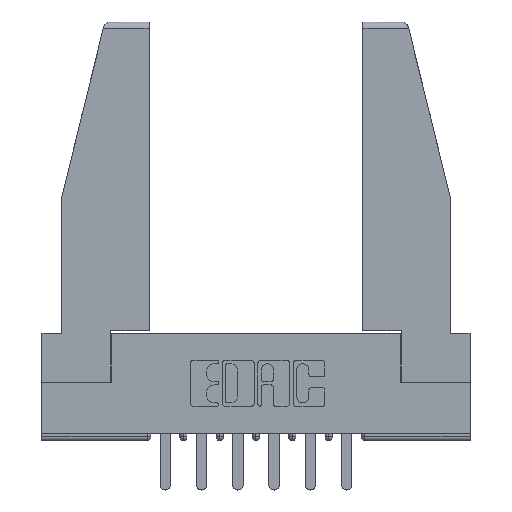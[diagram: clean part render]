
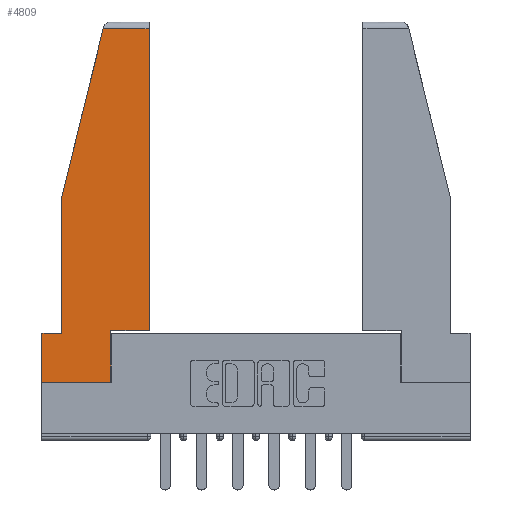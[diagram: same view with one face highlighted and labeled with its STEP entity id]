
A CAD part, top view. The second image highlights one B-rep face of the part: STEP entity #4809.
In plain terms, the highlighted planar face has unit normal (0, 0, 1).
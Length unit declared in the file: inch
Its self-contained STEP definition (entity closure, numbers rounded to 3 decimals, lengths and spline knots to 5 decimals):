
#142 = ORIENTED_EDGE ( 'NONE', *, *, #9193, .T. ) ;
#317 = EDGE_CURVE ( 'NONE', #8245, #10129, #10745, .T. ) ;
#431 = LINE ( 'NONE', #6958, #1872 ) ;
#1487 = VECTOR ( 'NONE', #5805, 39.37008 ) ;
#1565 = CARTESIAN_POINT ( 'NONE',  ( 0.2636, 1.52, 0. ) ) ;
#1872 = VECTOR ( 'NONE', #12044, 39.37008 ) ;
#1889 = VERTEX_POINT ( 'NONE', #7203 ) ;
#1959 = CARTESIAN_POINT ( 'NONE',  ( 0., 0.21, 0. ) ) ;
#2574 = EDGE_CURVE ( 'NONE', #11155, #6368, #4320, .T. ) ;
#2994 = CARTESIAN_POINT ( 'NONE',  ( 0., 0.21, 0. ) ) ;
#3124 = CARTESIAN_POINT ( 'NONE',  ( 0.461, 1.52, 0. ) ) ;
#3129 = CARTESIAN_POINT ( 'NONE',  ( 0., 0., 0. ) ) ;
#3348 = CARTESIAN_POINT ( 'NONE',  ( 0., 0., 0. ) ) ;
#3396 = ORIENTED_EDGE ( 'NONE', *, *, #2574, .T. ) ;
#3424 = EDGE_CURVE ( 'NONE', #10129, #6494, #5858, .T. ) ;
#3546 = CARTESIAN_POINT ( 'NONE',  ( 0., 1.52, 0. ) ) ;
#3784 = CARTESIAN_POINT ( 'NONE',  ( 0.086, 0.8, 0. ) ) ;
#3851 = EDGE_CURVE ( 'NONE', #9938, #8245, #10820, .T. ) ;
#3939 = LINE ( 'NONE', #2994, #7567 ) ;
#3979 = DIRECTION ( 'NONE',  ( 1., 0., 0. ) ) ;
#4041 = DIRECTION ( 'NONE',  ( 0., -1., 0. ) ) ;
#4129 = EDGE_LOOP ( 'NONE', ( #6269, #142, #6934, #8595, #9787, #11433, #3396, #6315, #10667 ) ) ;
#4194 = EDGE_CURVE ( 'NONE', #6368, #1889, #7581, .T. ) ;
#4320 = LINE ( 'NONE', #7460, #12112 ) ;
#4431 = VECTOR ( 'NONE', #6038, 39.37008 ) ;
#4789 = EDGE_CURVE ( 'NONE', #6494, #11155, #3939, .T. ) ;
#4809 = ADVANCED_FACE ( 'NONE', ( #7413 ), #6057, .T. ) ;
#5009 = DIRECTION ( 'NONE',  ( 0., 0., 1. ) ) ;
#5770 = LINE ( 'NONE', #9055, #6866 ) ;
#5805 = DIRECTION ( 'NONE',  ( 0., -1., 0. ) ) ;
#5858 = LINE ( 'NONE', #10623, #7448 ) ;
#5940 = DIRECTION ( 'NONE',  ( 0., 1., 0. ) ) ;
#6038 = DIRECTION ( 'NONE',  ( -0.239, -0.971, 0. ) ) ;
#6057 = PLANE ( 'NONE',  #11849 ) ;
#6083 = CARTESIAN_POINT ( 'NONE',  ( 0.271, 1.55, 0. ) ) ;
#6269 = ORIENTED_EDGE ( 'NONE', *, *, #8703, .T. ) ;
#6315 = ORIENTED_EDGE ( 'NONE', *, *, #4194, .T. ) ;
#6317 = LINE ( 'NONE', #3546, #11438 ) ;
#6368 = VERTEX_POINT ( 'NONE', #12519 ) ;
#6494 = VERTEX_POINT ( 'NONE', #1959 ) ;
#6523 = EDGE_CURVE ( 'NONE', #1889, #12700, #5770, .T. ) ;
#6866 = VECTOR ( 'NONE', #3979, 39.37008 ) ;
#6934 = ORIENTED_EDGE ( 'NONE', *, *, #3851, .T. ) ;
#6958 = CARTESIAN_POINT ( 'NONE',  ( 0.461, 0.223, 0. ) ) ;
#7203 = CARTESIAN_POINT ( 'NONE',  ( 0.297, 0.223, 0. ) ) ;
#7410 = CARTESIAN_POINT ( 'NONE',  ( 0.086, 0.8, 0. ) ) ;
#7413 = FACE_OUTER_BOUND ( 'NONE', #4129, .T. ) ;
#7448 = VECTOR ( 'NONE', #8515, 39.37008 ) ;
#7460 = CARTESIAN_POINT ( 'NONE',  ( 0., 0., 0. ) ) ;
#7567 = VECTOR ( 'NONE', #4041, 39.37008 ) ;
#7581 = LINE ( 'NONE', #7792, #9198 ) ;
#7792 = CARTESIAN_POINT ( 'NONE',  ( 0.297, 0., 0. ) ) ;
#8245 = VERTEX_POINT ( 'NONE', #7410 ) ;
#8515 = DIRECTION ( 'NONE',  ( -1., 0., 0. ) ) ;
#8595 = ORIENTED_EDGE ( 'NONE', *, *, #317, .T. ) ;
#8703 = EDGE_CURVE ( 'NONE', #12700, #11047, #431, .T. ) ;
#9055 = CARTESIAN_POINT ( 'NONE',  ( 0.297, 0.223, 0. ) ) ;
#9193 = EDGE_CURVE ( 'NONE', #11047, #9938, #6317, .T. ) ;
#9198 = VECTOR ( 'NONE', #5940, 39.37008 ) ;
#9551 = DIRECTION ( 'NONE',  ( 1., 0., 0. ) ) ;
#9604 = CARTESIAN_POINT ( 'NONE',  ( 0.461, 0.223, 0. ) ) ;
#9689 = CARTESIAN_POINT ( 'NONE',  ( 0.086, 0.21, 0. ) ) ;
#9787 = ORIENTED_EDGE ( 'NONE', *, *, #3424, .T. ) ;
#9938 = VERTEX_POINT ( 'NONE', #1565 ) ;
#10129 = VERTEX_POINT ( 'NONE', #9689 ) ;
#10623 = CARTESIAN_POINT ( 'NONE',  ( 0., 0.21, 0. ) ) ;
#10646 = DIRECTION ( 'NONE',  ( -1., 0., 0. ) ) ;
#10667 = ORIENTED_EDGE ( 'NONE', *, *, #6523, .T. ) ;
#10745 = LINE ( 'NONE', #3784, #1487 ) ;
#10820 = LINE ( 'NONE', #6083, #4431 ) ;
#11047 = VERTEX_POINT ( 'NONE', #3124 ) ;
#11155 = VERTEX_POINT ( 'NONE', #3348 ) ;
#11157 = DIRECTION ( 'NONE',  ( 1., 0., 0. ) ) ;
#11433 = ORIENTED_EDGE ( 'NONE', *, *, #4789, .T. ) ;
#11438 = VECTOR ( 'NONE', #10646, 39.37008 ) ;
#11849 = AXIS2_PLACEMENT_3D ( 'NONE', #3129, #5009, #11157 ) ;
#12044 = DIRECTION ( 'NONE',  ( 0., 1., 0. ) ) ;
#12112 = VECTOR ( 'NONE', #9551, 39.37008 ) ;
#12519 = CARTESIAN_POINT ( 'NONE',  ( 0.297, 0., 0. ) ) ;
#12700 = VERTEX_POINT ( 'NONE', #9604 ) ;
